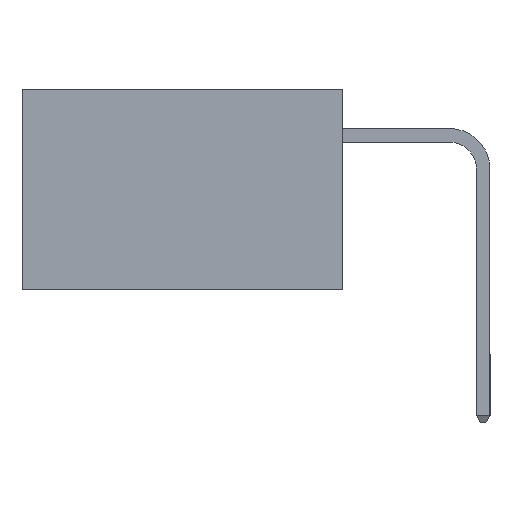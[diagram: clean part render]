
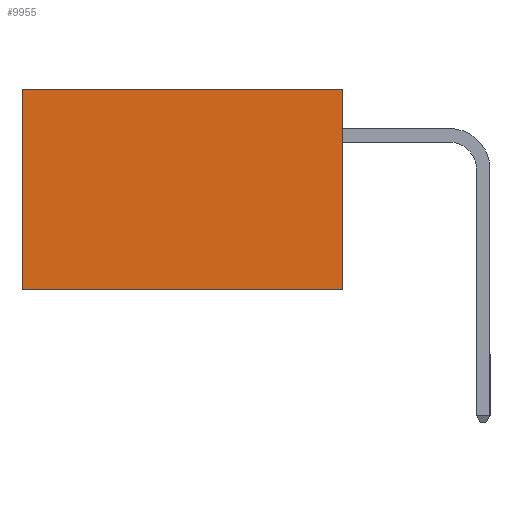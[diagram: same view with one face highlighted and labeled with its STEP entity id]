
A CAD part, left-side view. The second image highlights one B-rep face of the part: STEP entity #9955.
In plain terms, the highlighted planar face has unit normal (-1, 0, 0).
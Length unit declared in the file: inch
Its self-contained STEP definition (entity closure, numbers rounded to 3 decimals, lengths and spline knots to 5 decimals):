
#1190 = CARTESIAN_POINT ( 'NONE',  ( 0.277, 0., -0.37 ) ) ;
#1984 = CARTESIAN_POINT ( 'NONE',  ( 0.277, 0.59, -0.37 ) ) ;
#2179 = VERTEX_POINT ( 'NONE', #13384 ) ;
#2631 = LINE ( 'NONE', #9037, #14452 ) ;
#2649 = FACE_OUTER_BOUND ( 'NONE', #2819, .T. ) ;
#2819 = EDGE_LOOP ( 'NONE', ( #7258, #12759, #8352, #13885 ) ) ;
#3511 = EDGE_CURVE ( 'NONE', #5701, #8780, #13622, .T. ) ;
#3905 = DIRECTION ( 'NONE',  ( 1., 0., 0. ) ) ;
#3955 = CARTESIAN_POINT ( 'NONE',  ( 0.277, 0.59, -0.37 ) ) ;
#3974 = DIRECTION ( 'NONE',  ( 0., 0., -1. ) ) ;
#4163 = AXIS2_PLACEMENT_3D ( 'NONE', #10615, #3905, #11693 ) ;
#4487 = VECTOR ( 'NONE', #4728, 39.37008 ) ;
#4728 = DIRECTION ( 'NONE',  ( 0., 1., 0. ) ) ;
#4960 = VECTOR ( 'NONE', #3974, 39.37008 ) ;
#5064 = CARTESIAN_POINT ( 'NONE',  ( 0.277, 0., -0.37 ) ) ;
#5701 = VERTEX_POINT ( 'NONE', #8119 ) ;
#6453 = LINE ( 'NONE', #1190, #7120 ) ;
#6810 = EDGE_CURVE ( 'NONE', #2179, #8780, #7469, .T. ) ;
#7120 = VECTOR ( 'NONE', #9425, 39.37008 ) ;
#7258 = ORIENTED_EDGE ( 'NONE', *, *, #3511, .T. ) ;
#7469 = LINE ( 'NONE', #5064, #4487 ) ;
#8119 = CARTESIAN_POINT ( 'NONE',  ( 0.277, 0.59, 0. ) ) ;
#8334 = CARTESIAN_POINT ( 'NONE',  ( 0.277, 0., 0. ) ) ;
#8352 = ORIENTED_EDGE ( 'NONE', *, *, #9116, .F. ) ;
#8780 = VERTEX_POINT ( 'NONE', #1984 ) ;
#9037 = CARTESIAN_POINT ( 'NONE',  ( 0.277, 0., 0. ) ) ;
#9116 = EDGE_CURVE ( 'NONE', #10616, #2179, #6453, .T. ) ;
#9425 = DIRECTION ( 'NONE',  ( 0., 0., -1. ) ) ;
#9616 = EDGE_CURVE ( 'NONE', #10616, #5701, #2631, .T. ) ;
#9955 = ADVANCED_FACE ( 'NONE', ( #2649 ), #10563, .F. ) ;
#10120 = DIRECTION ( 'NONE',  ( 0., 1., 0. ) ) ;
#10563 = PLANE ( 'NONE',  #4163 ) ;
#10615 = CARTESIAN_POINT ( 'NONE',  ( 0.277, 0., -0.37 ) ) ;
#10616 = VERTEX_POINT ( 'NONE', #8334 ) ;
#11693 = DIRECTION ( 'NONE',  ( 0., 0., -1. ) ) ;
#12759 = ORIENTED_EDGE ( 'NONE', *, *, #6810, .F. ) ;
#13384 = CARTESIAN_POINT ( 'NONE',  ( 0.277, 0., -0.37 ) ) ;
#13622 = LINE ( 'NONE', #3955, #4960 ) ;
#13885 = ORIENTED_EDGE ( 'NONE', *, *, #9616, .T. ) ;
#14452 = VECTOR ( 'NONE', #10120, 39.37008 ) ;
